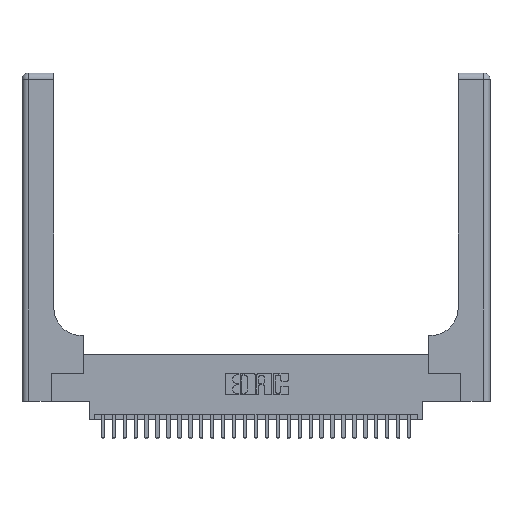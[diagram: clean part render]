
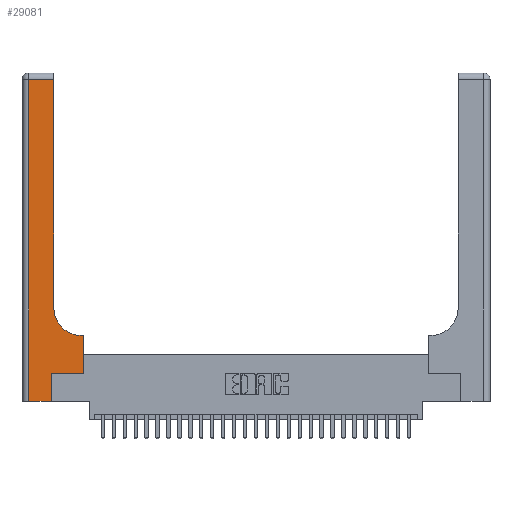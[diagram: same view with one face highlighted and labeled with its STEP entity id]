
A CAD part, top view. The second image highlights one B-rep face of the part: STEP entity #29081.
In plain terms, the highlighted planar face has unit normal (0, 0, 1).
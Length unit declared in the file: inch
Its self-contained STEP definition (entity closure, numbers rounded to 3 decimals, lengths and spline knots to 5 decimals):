
#1142 = VECTOR ( 'NONE', #18231, 39.37008 ) ;
#1409 = EDGE_CURVE ( 'NONE', #19862, #4643, #24070, .T. ) ;
#1445 = LINE ( 'NONE', #12384, #17759 ) ;
#1899 = LINE ( 'NONE', #20570, #1142 ) ;
#2214 = LINE ( 'NONE', #8667, #25376 ) ;
#2332 = ORIENTED_EDGE ( 'NONE', *, *, #7064, .T. ) ;
#3452 = ORIENTED_EDGE ( 'NONE', *, *, #11527, .T. ) ;
#3701 = CARTESIAN_POINT ( 'NONE',  ( 0.269, 0.25, 0.37 ) ) ;
#4159 = VECTOR ( 'NONE', #10214, 39.37008 ) ;
#4643 = VERTEX_POINT ( 'NONE', #14974 ) ;
#4951 = LINE ( 'NONE', #5391, #22695 ) ;
#5391 = CARTESIAN_POINT ( 'NONE',  ( 0.269, 0., 0.37 ) ) ;
#5585 = EDGE_CURVE ( 'NONE', #4643, #23265, #23493, .T. ) ;
#5629 = CARTESIAN_POINT ( 'NONE',  ( 0.5415, 0.6, 0.37 ) ) ;
#5967 = VERTEX_POINT ( 'NONE', #3701 ) ;
#6459 = CARTESIAN_POINT ( 'NONE',  ( 0., 2.94, 0.37 ) ) ;
#7064 = EDGE_CURVE ( 'NONE', #23265, #8234, #14433, .T. ) ;
#7726 = DIRECTION ( 'NONE',  ( 0., 1., 0. ) ) ;
#7866 = CARTESIAN_POINT ( 'NONE',  ( 0.06, 3., 0.37 ) ) ;
#8234 = VERTEX_POINT ( 'NONE', #13285 ) ;
#8279 = VECTOR ( 'NONE', #22664, 39.37008 ) ;
#8667 = CARTESIAN_POINT ( 'NONE',  ( 0.5585, 0.25, 0.37 ) ) ;
#10214 = DIRECTION ( 'NONE',  ( 0., -1., 0. ) ) ;
#10310 = LINE ( 'NONE', #7866, #4159 ) ;
#10341 = ORIENTED_EDGE ( 'NONE', *, *, #12101, .T. ) ;
#11136 = PLANE ( 'NONE',  #13940 ) ;
#11209 = VECTOR ( 'NONE', #11313, 39.37008 ) ;
#11313 = DIRECTION ( 'NONE',  ( 0., 1., 0. ) ) ;
#11527 = EDGE_CURVE ( 'NONE', #20855, #24308, #2214, .T. ) ;
#11786 = ORIENTED_EDGE ( 'NONE', *, *, #1409, .T. ) ;
#12101 = EDGE_CURVE ( 'NONE', #24308, #19862, #1445, .T. ) ;
#12384 = CARTESIAN_POINT ( 'NONE',  ( 0.2915, 0.6, 0.37 ) ) ;
#12482 = ORIENTED_EDGE ( 'NONE', *, *, #5585, .T. ) ;
#12497 = CARTESIAN_POINT ( 'NONE',  ( 0.5585, 0.6, 0.37 ) ) ;
#12845 = ORIENTED_EDGE ( 'NONE', *, *, #22283, .T. ) ;
#13285 = CARTESIAN_POINT ( 'NONE',  ( 0.06, 2.94, 0.37 ) ) ;
#13433 = DIRECTION ( 'NONE',  ( -1., 0., 0. ) ) ;
#13521 = CARTESIAN_POINT ( 'NONE',  ( 0.5415, 0.85, 0.37 ) ) ;
#13703 = CARTESIAN_POINT ( 'NONE',  ( 0.06, 0., 0.37 ) ) ;
#13940 = AXIS2_PLACEMENT_3D ( 'NONE', #17998, #27284, #13433 ) ;
#14303 = ORIENTED_EDGE ( 'NONE', *, *, #23428, .T. ) ;
#14433 = LINE ( 'NONE', #6459, #8279 ) ;
#14974 = CARTESIAN_POINT ( 'NONE',  ( 0.2915, 0.85, 0.37 ) ) ;
#15009 = FACE_OUTER_BOUND ( 'NONE', #28377, .T. ) ;
#15847 = DIRECTION ( 'NONE',  ( 1., 0., 0. ) ) ;
#16034 = AXIS2_PLACEMENT_3D ( 'NONE', #13521, #29667, #15847 ) ;
#16093 = CARTESIAN_POINT ( 'NONE',  ( 0.269, 0., 0.37 ) ) ;
#16097 = LINE ( 'NONE', #24452, #17553 ) ;
#16100 = ORIENTED_EDGE ( 'NONE', *, *, #23653, .T. ) ;
#16305 = CARTESIAN_POINT ( 'NONE',  ( 0.5585, 0.25, 0.37 ) ) ;
#17553 = VECTOR ( 'NONE', #26759, 39.37008 ) ;
#17759 = VECTOR ( 'NONE', #26194, 39.37008 ) ;
#17998 = CARTESIAN_POINT ( 'NONE',  ( 0., 3., 0.37 ) ) ;
#18231 = DIRECTION ( 'NONE',  ( 1., 0., 0. ) ) ;
#18920 = CARTESIAN_POINT ( 'NONE',  ( 0.2915, 2.94, 0.37 ) ) ;
#18921 = EDGE_CURVE ( 'NONE', #22130, #26707, #1899, .T. ) ;
#19862 = VERTEX_POINT ( 'NONE', #5629 ) ;
#20524 = CARTESIAN_POINT ( 'NONE',  ( 0.2915, 3., 0.37 ) ) ;
#20570 = CARTESIAN_POINT ( 'NONE',  ( 0., 0., 0.37 ) ) ;
#20855 = VERTEX_POINT ( 'NONE', #16305 ) ;
#22130 = VERTEX_POINT ( 'NONE', #13703 ) ;
#22283 = EDGE_CURVE ( 'NONE', #26707, #5967, #4951, .T. ) ;
#22664 = DIRECTION ( 'NONE',  ( -1., 0., 0. ) ) ;
#22695 = VECTOR ( 'NONE', #7726, 39.37008 ) ;
#23265 = VERTEX_POINT ( 'NONE', #18920 ) ;
#23428 = EDGE_CURVE ( 'NONE', #5967, #20855, #16097, .T. ) ;
#23493 = LINE ( 'NONE', #20524, #11209 ) ;
#23653 = EDGE_CURVE ( 'NONE', #8234, #22130, #10310, .T. ) ;
#23723 = ORIENTED_EDGE ( 'NONE', *, *, #18921, .T. ) ;
#24070 = CIRCLE ( 'NONE', #16034, 0.25 ) ;
#24308 = VERTEX_POINT ( 'NONE', #12497 ) ;
#24452 = CARTESIAN_POINT ( 'NONE',  ( 0.269, 0.25, 0.37 ) ) ;
#25376 = VECTOR ( 'NONE', #27262, 39.37008 ) ;
#26194 = DIRECTION ( 'NONE',  ( -1., 0., 0. ) ) ;
#26707 = VERTEX_POINT ( 'NONE', #16093 ) ;
#26759 = DIRECTION ( 'NONE',  ( 1., 0., 0. ) ) ;
#27262 = DIRECTION ( 'NONE',  ( 0., 1., 0. ) ) ;
#27284 = DIRECTION ( 'NONE',  ( 0., 0., -1. ) ) ;
#28377 = EDGE_LOOP ( 'NONE', ( #12482, #2332, #16100, #23723, #12845, #14303, #3452, #10341, #11786 ) ) ;
#29081 = ADVANCED_FACE ( 'NONE', ( #15009 ), #11136, .F. ) ;
#29667 = DIRECTION ( 'NONE',  ( 0., 0., -1. ) ) ;
